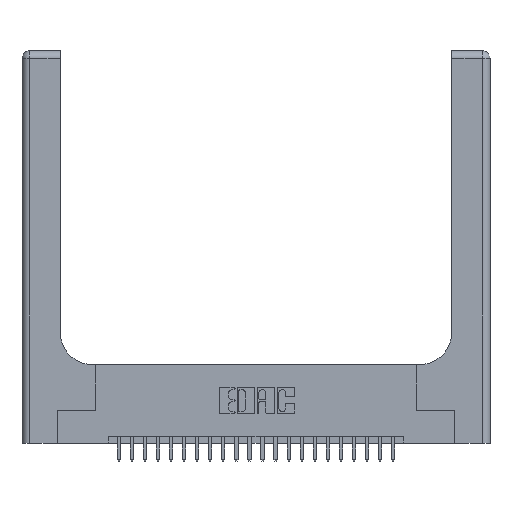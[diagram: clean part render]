
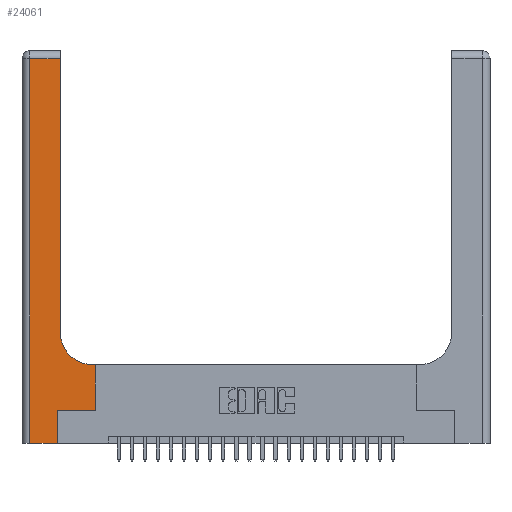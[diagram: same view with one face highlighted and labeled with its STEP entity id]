
A CAD part, top view. The second image highlights one B-rep face of the part: STEP entity #24061.
In plain terms, the highlighted planar face has unit normal (0, 0, 1).
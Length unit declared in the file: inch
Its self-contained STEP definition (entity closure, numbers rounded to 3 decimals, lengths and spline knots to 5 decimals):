
#446 = CARTESIAN_POINT ( 'NONE',  ( 0.269, 0., 0.37 ) ) ;
#610 = VECTOR ( 'NONE', #11721, 39.37008 ) ;
#924 = LINE ( 'NONE', #15013, #19793 ) ;
#988 = EDGE_CURVE ( 'NONE', #13960, #10142, #9771, .T. ) ;
#1022 = DIRECTION ( 'NONE',  ( 0., 1., 0. ) ) ;
#1565 = DIRECTION ( 'NONE',  ( -1., 0., 0. ) ) ;
#2061 = VECTOR ( 'NONE', #1022, 39.37008 ) ;
#2344 = CARTESIAN_POINT ( 'NONE',  ( 0.5585, 0.25, 0.37 ) ) ;
#2385 = DIRECTION ( 'NONE',  ( 0., 0., -1. ) ) ;
#2682 = CARTESIAN_POINT ( 'NONE',  ( 0.2915, 2.94, 0.37 ) ) ;
#3171 = VERTEX_POINT ( 'NONE', #20084 ) ;
#3484 = EDGE_CURVE ( 'NONE', #14272, #13960, #23752, .T. ) ;
#3763 = VERTEX_POINT ( 'NONE', #446 ) ;
#3765 = ORIENTED_EDGE ( 'NONE', *, *, #6194, .T. ) ;
#4924 = DIRECTION ( 'NONE',  ( 0., 0., -1. ) ) ;
#5720 = CARTESIAN_POINT ( 'NONE',  ( 0.2915, 0.6, 0.37 ) ) ;
#5931 = EDGE_CURVE ( 'NONE', #17402, #3171, #13020, .T. ) ;
#6194 = EDGE_CURVE ( 'NONE', #3171, #8489, #6309, .T. ) ;
#6309 = LINE ( 'NONE', #5720, #10851 ) ;
#6651 = LINE ( 'NONE', #8138, #15782 ) ;
#6682 = ORIENTED_EDGE ( 'NONE', *, *, #988, .T. ) ;
#7598 = EDGE_CURVE ( 'NONE', #10142, #3763, #17798, .T. ) ;
#7670 = DIRECTION ( 'NONE',  ( -1., 0., 0. ) ) ;
#8138 = CARTESIAN_POINT ( 'NONE',  ( 0.2915, 3., 0.37 ) ) ;
#8489 = VERTEX_POINT ( 'NONE', #16512 ) ;
#8795 = ORIENTED_EDGE ( 'NONE', *, *, #3484, .T. ) ;
#9399 = CARTESIAN_POINT ( 'NONE',  ( 0., 2.94, 0.37 ) ) ;
#9557 = VERTEX_POINT ( 'NONE', #23738 ) ;
#9653 = ORIENTED_EDGE ( 'NONE', *, *, #17395, .T. ) ;
#9678 = CARTESIAN_POINT ( 'NONE',  ( 0., 0., 0.37 ) ) ;
#9771 = LINE ( 'NONE', #11320, #610 ) ;
#9801 = ORIENTED_EDGE ( 'NONE', *, *, #23212, .T. ) ;
#10142 = VERTEX_POINT ( 'NONE', #12917 ) ;
#10678 = ORIENTED_EDGE ( 'NONE', *, *, #19106, .T. ) ;
#10718 = CARTESIAN_POINT ( 'NONE',  ( 0.5585, 0.25, 0.37 ) ) ;
#10846 = AXIS2_PLACEMENT_3D ( 'NONE', #16584, #4924, #18509 ) ;
#10851 = VECTOR ( 'NONE', #7670, 39.37008 ) ;
#11320 = CARTESIAN_POINT ( 'NONE',  ( 0.06, 3., 0.37 ) ) ;
#11631 = DIRECTION ( 'NONE',  ( 1., 0., 0. ) ) ;
#11721 = DIRECTION ( 'NONE',  ( 0., -1., 0. ) ) ;
#12071 = DIRECTION ( 'NONE',  ( 0., 1., 0. ) ) ;
#12624 = VECTOR ( 'NONE', #11631, 39.37008 ) ;
#12917 = CARTESIAN_POINT ( 'NONE',  ( 0.06, 0., 0.37 ) ) ;
#13020 = LINE ( 'NONE', #10718, #2061 ) ;
#13474 = VECTOR ( 'NONE', #1565, 39.37008 ) ;
#13960 = VERTEX_POINT ( 'NONE', #20943 ) ;
#14033 = CARTESIAN_POINT ( 'NONE',  ( 0., 3., 0.37 ) ) ;
#14187 = VECTOR ( 'NONE', #12071, 39.37008 ) ;
#14272 = VERTEX_POINT ( 'NONE', #2682 ) ;
#15013 = CARTESIAN_POINT ( 'NONE',  ( 0.269, 0.25, 0.37 ) ) ;
#15782 = VECTOR ( 'NONE', #21590, 39.37008 ) ;
#16006 = DIRECTION ( 'NONE',  ( -1., 0., 0. ) ) ;
#16309 = EDGE_CURVE ( 'NONE', #8489, #9557, #21263, .T. ) ;
#16512 = CARTESIAN_POINT ( 'NONE',  ( 0.5415, 0.6, 0.37 ) ) ;
#16584 = CARTESIAN_POINT ( 'NONE',  ( 0.5415, 0.85, 0.37 ) ) ;
#17395 = EDGE_CURVE ( 'NONE', #9557, #14272, #6651, .T. ) ;
#17402 = VERTEX_POINT ( 'NONE', #2344 ) ;
#17798 = LINE ( 'NONE', #9678, #12624 ) ;
#17818 = CARTESIAN_POINT ( 'NONE',  ( 0.269, 0.25, 0.37 ) ) ;
#18509 = DIRECTION ( 'NONE',  ( 1., 0., 0. ) ) ;
#18712 = LINE ( 'NONE', #23661, #14187 ) ;
#19106 = EDGE_CURVE ( 'NONE', #3763, #21596, #18712, .T. ) ;
#19785 = PLANE ( 'NONE',  #21361 ) ;
#19793 = VECTOR ( 'NONE', #24640, 39.37008 ) ;
#20084 = CARTESIAN_POINT ( 'NONE',  ( 0.5585, 0.6, 0.37 ) ) ;
#20326 = FACE_OUTER_BOUND ( 'NONE', #24350, .T. ) ;
#20727 = ORIENTED_EDGE ( 'NONE', *, *, #5931, .T. ) ;
#20943 = CARTESIAN_POINT ( 'NONE',  ( 0.06, 2.94, 0.37 ) ) ;
#21222 = ORIENTED_EDGE ( 'NONE', *, *, #7598, .T. ) ;
#21263 = CIRCLE ( 'NONE', #10846, 0.25 ) ;
#21361 = AXIS2_PLACEMENT_3D ( 'NONE', #14033, #2385, #16006 ) ;
#21590 = DIRECTION ( 'NONE',  ( 0., 1., 0. ) ) ;
#21596 = VERTEX_POINT ( 'NONE', #17818 ) ;
#23212 = EDGE_CURVE ( 'NONE', #21596, #17402, #924, .T. ) ;
#23529 = ORIENTED_EDGE ( 'NONE', *, *, #16309, .T. ) ;
#23661 = CARTESIAN_POINT ( 'NONE',  ( 0.269, 0., 0.37 ) ) ;
#23738 = CARTESIAN_POINT ( 'NONE',  ( 0.2915, 0.85, 0.37 ) ) ;
#23752 = LINE ( 'NONE', #9399, #13474 ) ;
#24061 = ADVANCED_FACE ( 'NONE', ( #20326 ), #19785, .F. ) ;
#24350 = EDGE_LOOP ( 'NONE', ( #9653, #8795, #6682, #21222, #10678, #9801, #20727, #3765, #23529 ) ) ;
#24640 = DIRECTION ( 'NONE',  ( 1., 0., 0. ) ) ;
